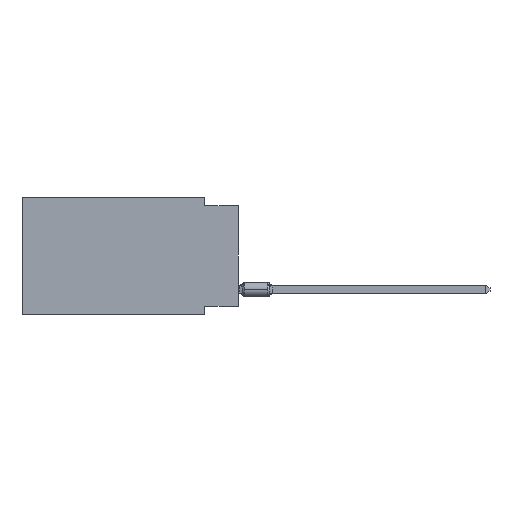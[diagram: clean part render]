
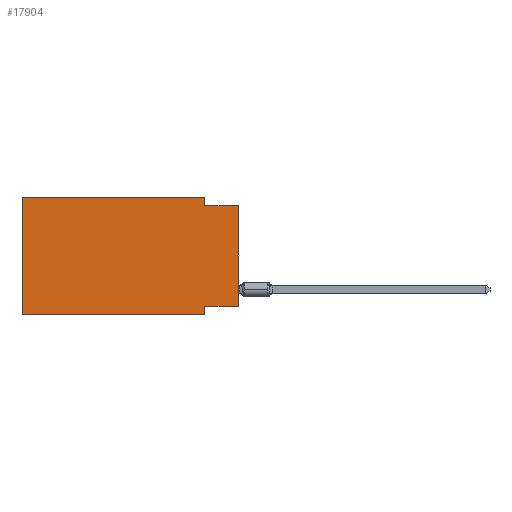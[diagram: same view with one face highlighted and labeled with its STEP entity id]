
A CAD part, left-side view. The second image highlights one B-rep face of the part: STEP entity #17904.
In plain terms, the highlighted planar face has unit normal (-1, 0, 0).
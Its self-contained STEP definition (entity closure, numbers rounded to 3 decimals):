
#1219 = LINE ( 'NONE', #2813, #4210 ) ;
#1402 = CARTESIAN_POINT ( 'NONE',  ( 0., 0., 0. ) ) ;
#1461 = VERTEX_POINT ( 'NONE', #6670 ) ;
#1653 = VECTOR ( 'NONE', #2990, 1000. ) ;
#2813 = CARTESIAN_POINT ( 'NONE',  ( 0., 16.383, -8.89 ) ) ;
#2990 = DIRECTION ( 'NONE',  ( 0., 1., 0. ) ) ;
#3297 = FACE_OUTER_BOUND ( 'NONE', #11329, .T. ) ;
#3401 = LINE ( 'NONE', #9730, #8195 ) ;
#3773 = VECTOR ( 'NONE', #4482, 1000. ) ;
#4210 = VECTOR ( 'NONE', #19200, 1000. ) ;
#4329 = ORIENTED_EDGE ( 'NONE', *, *, #17257, .T. ) ;
#4482 = DIRECTION ( 'NONE',  ( 0., 0., -1. ) ) ;
#4783 = CARTESIAN_POINT ( 'NONE',  ( 0., 0., -0.635 ) ) ;
#5192 = EDGE_CURVE ( 'NONE', #17796, #11309, #1219, .T. ) ;
#5425 = ORIENTED_EDGE ( 'NONE', *, *, #5192, .T. ) ;
#6084 = CARTESIAN_POINT ( 'NONE',  ( 0., 2.54, 0. ) ) ;
#6188 = CARTESIAN_POINT ( 'NONE',  ( 0., 2.54, -0.635 ) ) ;
#6670 = CARTESIAN_POINT ( 'NONE',  ( 0., 2.54, -8.255 ) ) ;
#7319 = ORIENTED_EDGE ( 'NONE', *, *, #11269, .F. ) ;
#7595 = CARTESIAN_POINT ( 'NONE',  ( 0., 2.54, -8.89 ) ) ;
#7807 = CARTESIAN_POINT ( 'NONE',  ( 0., 2.54, -8.89 ) ) ;
#7926 = LINE ( 'NONE', #11147, #11123 ) ;
#8130 = CARTESIAN_POINT ( 'NONE',  ( 0., 0., -8.255 ) ) ;
#8195 = VECTOR ( 'NONE', #8222, 1000. ) ;
#8222 = DIRECTION ( 'NONE',  ( 0., 0., 1. ) ) ;
#8263 = CARTESIAN_POINT ( 'NONE',  ( 0., 0., -0.635 ) ) ;
#9730 = CARTESIAN_POINT ( 'NONE',  ( 0., 16.383, 0. ) ) ;
#9931 = VERTEX_POINT ( 'NONE', #18511 ) ;
#10147 = VERTEX_POINT ( 'NONE', #6188 ) ;
#10447 = VERTEX_POINT ( 'NONE', #4783 ) ;
#10555 = DIRECTION ( 'NONE',  ( 1., 0., 0. ) ) ;
#10601 = DIRECTION ( 'NONE',  ( 0., 0., -1. ) ) ;
#10937 = CARTESIAN_POINT ( 'NONE',  ( 0., 0., -8.255 ) ) ;
#11123 = VECTOR ( 'NONE', #13057, 1000. ) ;
#11147 = CARTESIAN_POINT ( 'NONE',  ( 0., 16.383, 0. ) ) ;
#11269 = EDGE_CURVE ( 'NONE', #9931, #10147, #20777, .T. ) ;
#11309 = VERTEX_POINT ( 'NONE', #7807 ) ;
#11329 = EDGE_LOOP ( 'NONE', ( #4329, #16608, #7319, #11486, #20892, #5425, #16667, #19482 ) ) ;
#11354 = EDGE_CURVE ( 'NONE', #14672, #1461, #17973, .T. ) ;
#11486 = ORIENTED_EDGE ( 'NONE', *, *, #13612, .F. ) ;
#11929 = EDGE_CURVE ( 'NONE', #10147, #10447, #17686, .T. ) ;
#12877 = DIRECTION ( 'NONE',  ( 0., -1., 0. ) ) ;
#13057 = DIRECTION ( 'NONE',  ( 0., -1., 0. ) ) ;
#13509 = EDGE_CURVE ( 'NONE', #1461, #11309, #19175, .T. ) ;
#13552 = CARTESIAN_POINT ( 'NONE',  ( 0., 16.383, 0. ) ) ;
#13612 = EDGE_CURVE ( 'NONE', #15361, #9931, #7926, .T. ) ;
#14672 = VERTEX_POINT ( 'NONE', #10937 ) ;
#15361 = VERTEX_POINT ( 'NONE', #20945 ) ;
#16031 = AXIS2_PLACEMENT_3D ( 'NONE', #13552, #10555, #18272 ) ;
#16608 = ORIENTED_EDGE ( 'NONE', *, *, #11929, .F. ) ;
#16667 = ORIENTED_EDGE ( 'NONE', *, *, #13509, .F. ) ;
#17257 = EDGE_CURVE ( 'NONE', #14672, #10447, #19073, .T. ) ;
#17563 = DIRECTION ( 'NONE',  ( 0., 0., 1. ) ) ;
#17603 = VECTOR ( 'NONE', #10601, 1000. ) ;
#17686 = LINE ( 'NONE', #8263, #20477 ) ;
#17796 = VERTEX_POINT ( 'NONE', #19590 ) ;
#17904 = ADVANCED_FACE ( 'NONE', ( #3297 ), #18483, .F. ) ;
#17973 = LINE ( 'NONE', #8130, #1653 ) ;
#18272 = DIRECTION ( 'NONE',  ( 0., 0., -1. ) ) ;
#18483 = PLANE ( 'NONE',  #16031 ) ;
#18511 = CARTESIAN_POINT ( 'NONE',  ( 0., 2.54, 0. ) ) ;
#18931 = EDGE_CURVE ( 'NONE', #17796, #15361, #3401, .T. ) ;
#19073 = LINE ( 'NONE', #1402, #21164 ) ;
#19175 = LINE ( 'NONE', #7595, #17603 ) ;
#19200 = DIRECTION ( 'NONE',  ( 0., -1., 0. ) ) ;
#19482 = ORIENTED_EDGE ( 'NONE', *, *, #11354, .F. ) ;
#19590 = CARTESIAN_POINT ( 'NONE',  ( 0., 16.383, -8.89 ) ) ;
#20477 = VECTOR ( 'NONE', #12877, 1000. ) ;
#20777 = LINE ( 'NONE', #6084, #3773 ) ;
#20892 = ORIENTED_EDGE ( 'NONE', *, *, #18931, .F. ) ;
#20945 = CARTESIAN_POINT ( 'NONE',  ( 0., 16.383, 0. ) ) ;
#21164 = VECTOR ( 'NONE', #17563, 1000. ) ;
